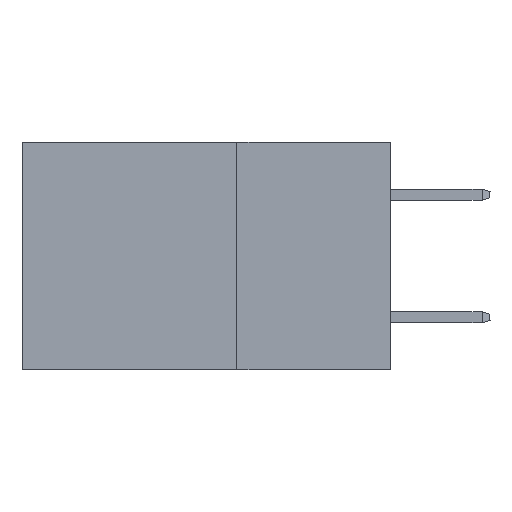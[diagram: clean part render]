
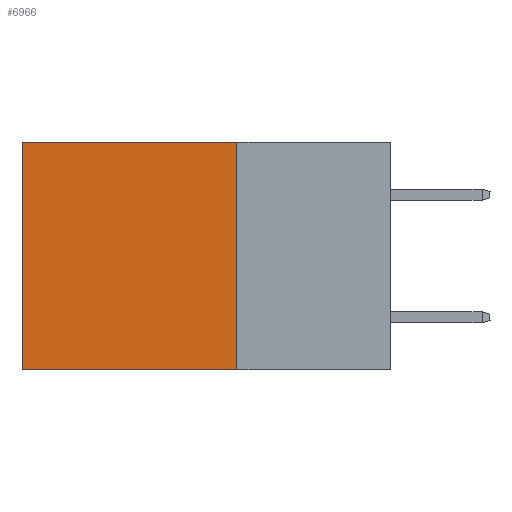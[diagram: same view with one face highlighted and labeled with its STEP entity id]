
A CAD part, left-side view. The second image highlights one B-rep face of the part: STEP entity #6966.
In plain terms, the highlighted planar face has unit normal (-1, 0, 0).
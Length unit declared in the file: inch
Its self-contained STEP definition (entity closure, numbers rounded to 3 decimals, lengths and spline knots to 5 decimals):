
#1535 = CARTESIAN_POINT ( 'NONE',  ( 0.2875, 0.25, -0.37 ) ) ;
#2043 = ORIENTED_EDGE ( 'NONE', *, *, #9272, .F. ) ;
#3282 = DIRECTION ( 'NONE',  ( 0., 0., -1. ) ) ;
#3459 = ORIENTED_EDGE ( 'NONE', *, *, #20568, .F. ) ;
#4497 = LINE ( 'NONE', #23609, #9918 ) ;
#4745 = LINE ( 'NONE', #22419, #20420 ) ;
#4795 = VECTOR ( 'NONE', #5777, 39.37008 ) ;
#5777 = DIRECTION ( 'NONE',  ( 0., 1., 0. ) ) ;
#6966 = ADVANCED_FACE ( 'NONE', ( #8249 ), #31733, .F. ) ;
#8249 = FACE_OUTER_BOUND ( 'NONE', #23504, .T. ) ;
#8487 = EDGE_CURVE ( 'NONE', #18196, #22213, #31938, .T. ) ;
#9272 = EDGE_CURVE ( 'NONE', #15024, #32200, #4745, .T. ) ;
#9858 = ORIENTED_EDGE ( 'NONE', *, *, #8487, .T. ) ;
#9878 = VECTOR ( 'NONE', #12715, 39.37008 ) ;
#9918 = VECTOR ( 'NONE', #31500, 39.37008 ) ;
#12715 = DIRECTION ( 'NONE',  ( 0., 0., -1. ) ) ;
#13846 = CARTESIAN_POINT ( 'NONE',  ( 0.2875, 0.6, 0. ) ) ;
#15024 = VERTEX_POINT ( 'NONE', #1535 ) ;
#16554 = CARTESIAN_POINT ( 'NONE',  ( 0.2875, 0.25, 0. ) ) ;
#18196 = VERTEX_POINT ( 'NONE', #21444 ) ;
#19178 = DIRECTION ( 'NONE',  ( 1., 0., 0. ) ) ;
#20420 = VECTOR ( 'NONE', #25054, 39.37008 ) ;
#20568 = EDGE_CURVE ( 'NONE', #18196, #15024, #31605, .T. ) ;
#20647 = ORIENTED_EDGE ( 'NONE', *, *, #26559, .T. ) ;
#20670 = CARTESIAN_POINT ( 'NONE',  ( 0.2875, 0.6, -0.37 ) ) ;
#21444 = CARTESIAN_POINT ( 'NONE',  ( 0.2875, 0.25, 0. ) ) ;
#21556 = CARTESIAN_POINT ( 'NONE',  ( 0.2875, 0.25, 0. ) ) ;
#22213 = VERTEX_POINT ( 'NONE', #13846 ) ;
#22419 = CARTESIAN_POINT ( 'NONE',  ( 0.2875, 0.25, -0.37 ) ) ;
#23504 = EDGE_LOOP ( 'NONE', ( #20647, #2043, #3459, #9858 ) ) ;
#23609 = CARTESIAN_POINT ( 'NONE',  ( 0.2875, 0.6, 0. ) ) ;
#25054 = DIRECTION ( 'NONE',  ( 0., 1., 0. ) ) ;
#26559 = EDGE_CURVE ( 'NONE', #22213, #32200, #4497, .T. ) ;
#30061 = AXIS2_PLACEMENT_3D ( 'NONE', #16554, #19178, #3282 ) ;
#31027 = CARTESIAN_POINT ( 'NONE',  ( 0.2875, 0.25, 0. ) ) ;
#31500 = DIRECTION ( 'NONE',  ( 0., 0., -1. ) ) ;
#31605 = LINE ( 'NONE', #31027, #9878 ) ;
#31733 = PLANE ( 'NONE',  #30061 ) ;
#31938 = LINE ( 'NONE', #21556, #4795 ) ;
#32200 = VERTEX_POINT ( 'NONE', #20670 ) ;
